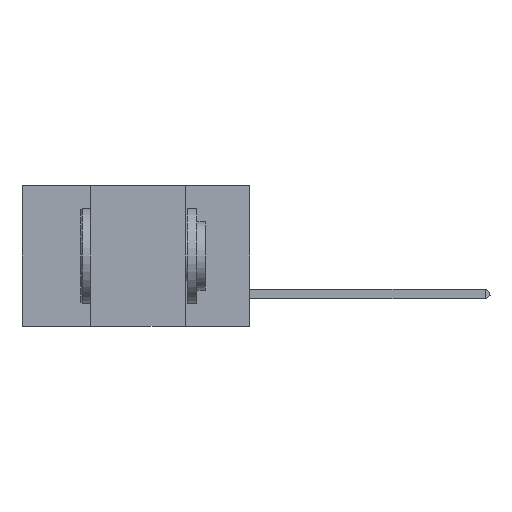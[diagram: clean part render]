
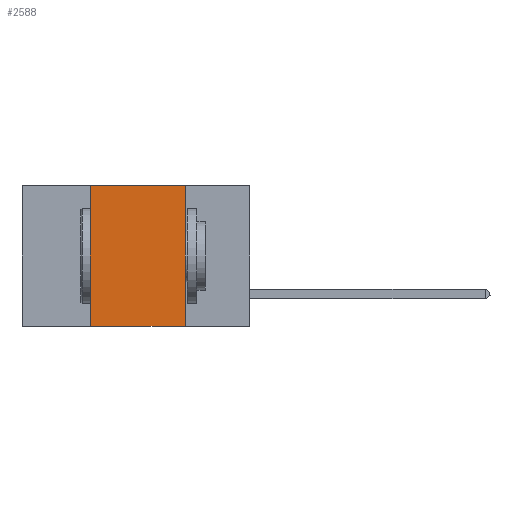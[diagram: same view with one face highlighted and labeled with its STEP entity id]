
A CAD part, left-side view. The second image highlights one B-rep face of the part: STEP entity #2588.
In plain terms, the highlighted planar face has unit normal (-1, 0, 0).
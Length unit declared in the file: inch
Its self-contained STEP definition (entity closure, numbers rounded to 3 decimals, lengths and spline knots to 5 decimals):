
#27 = FACE_OUTER_BOUND ( 'NONE', #6851, .T. ) ;
#65 = DIRECTION ( 'NONE',  ( 0., -1., 0. ) ) ;
#331 = PLANE ( 'NONE',  #1882 ) ;
#1205 = VERTEX_POINT ( 'NONE', #9468 ) ;
#1400 = VECTOR ( 'NONE', #6934, 39.37008 ) ;
#1765 = VERTEX_POINT ( 'NONE', #8379 ) ;
#1882 = AXIS2_PLACEMENT_3D ( 'NONE', #9275, #6179, #11085 ) ;
#1891 = CARTESIAN_POINT ( 'NONE',  ( 0., 0.17, -0.37 ) ) ;
#2467 = EDGE_CURVE ( 'NONE', #1765, #9751, #5189, .T. ) ;
#2588 = ADVANCED_FACE ( 'NONE', ( #27 ), #331, .F. ) ;
#2891 = VECTOR ( 'NONE', #65, 39.37008 ) ;
#3080 = DIRECTION ( 'NONE',  ( 0., 0., 1. ) ) ;
#3553 = CARTESIAN_POINT ( 'NONE',  ( 0., 0.17, 0. ) ) ;
#3725 = EDGE_CURVE ( 'NONE', #1205, #4825, #7741, .T. ) ;
#3769 = ORIENTED_EDGE ( 'NONE', *, *, #6454, .F. ) ;
#3822 = LINE ( 'NONE', #11803, #9629 ) ;
#4011 = LINE ( 'NONE', #11790, #1400 ) ;
#4825 = VERTEX_POINT ( 'NONE', #3553 ) ;
#4968 = ORIENTED_EDGE ( 'NONE', *, *, #7914, .F. ) ;
#5155 = VECTOR ( 'NONE', #7379, 39.37008 ) ;
#5189 = LINE ( 'NONE', #5824, #2891 ) ;
#5824 = CARTESIAN_POINT ( 'NONE',  ( 0., 0.6, -0.37 ) ) ;
#6148 = ORIENTED_EDGE ( 'NONE', *, *, #2467, .T. ) ;
#6179 = DIRECTION ( 'NONE',  ( 1., 0., 0. ) ) ;
#6391 = CARTESIAN_POINT ( 'NONE',  ( 0., 0.6, 0. ) ) ;
#6454 = EDGE_CURVE ( 'NONE', #4825, #9751, #4011, .T. ) ;
#6851 = EDGE_LOOP ( 'NONE', ( #3769, #6942, #4968, #6148 ) ) ;
#6934 = DIRECTION ( 'NONE',  ( 0., 0., -1. ) ) ;
#6942 = ORIENTED_EDGE ( 'NONE', *, *, #3725, .F. ) ;
#7379 = DIRECTION ( 'NONE',  ( 0., -1., 0. ) ) ;
#7741 = LINE ( 'NONE', #6391, #5155 ) ;
#7914 = EDGE_CURVE ( 'NONE', #1765, #1205, #3822, .T. ) ;
#8379 = CARTESIAN_POINT ( 'NONE',  ( 0., 0.42, -0.37 ) ) ;
#9275 = CARTESIAN_POINT ( 'NONE',  ( 0., 0.6, 0. ) ) ;
#9468 = CARTESIAN_POINT ( 'NONE',  ( 0., 0.42, 0. ) ) ;
#9629 = VECTOR ( 'NONE', #3080, 39.37008 ) ;
#9751 = VERTEX_POINT ( 'NONE', #1891 ) ;
#11085 = DIRECTION ( 'NONE',  ( 0., 0., -1. ) ) ;
#11790 = CARTESIAN_POINT ( 'NONE',  ( 0., 0.17, 0. ) ) ;
#11803 = CARTESIAN_POINT ( 'NONE',  ( 0., 0.42, 0. ) ) ;
